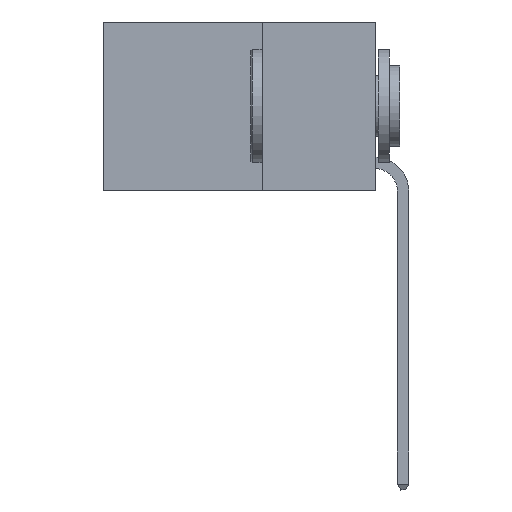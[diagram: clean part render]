
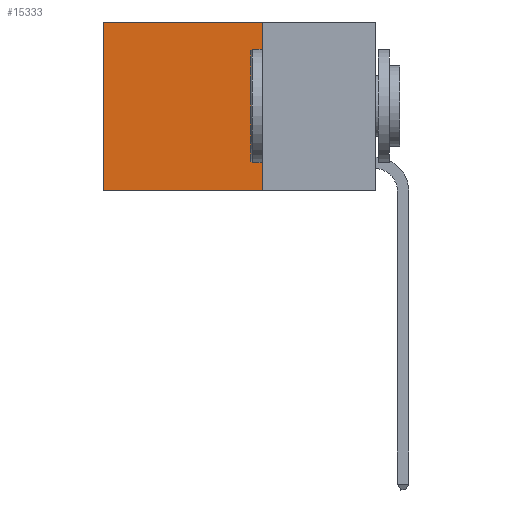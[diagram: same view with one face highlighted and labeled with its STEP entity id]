
A CAD part, left-side view. The second image highlights one B-rep face of the part: STEP entity #15333.
In plain terms, the highlighted planar face has unit normal (-1, 0, 0).
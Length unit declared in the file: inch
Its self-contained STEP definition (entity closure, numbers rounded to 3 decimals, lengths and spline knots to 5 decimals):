
#120 = EDGE_CURVE ( 'NONE', #6034, #5450, #17136, .T. ) ;
#121 = CARTESIAN_POINT ( 'NONE',  ( 0.2625, 0.25, 0. ) ) ;
#927 = CARTESIAN_POINT ( 'NONE',  ( 0.2625, 0.6, 0. ) ) ;
#1269 = EDGE_CURVE ( 'NONE', #15611, #5450, #10106, .T. ) ;
#1338 = EDGE_LOOP ( 'NONE', ( #2834, #15156, #6869, #9837 ) ) ;
#2278 = DIRECTION ( 'NONE',  ( 0., 0., -1. ) ) ;
#2834 = ORIENTED_EDGE ( 'NONE', *, *, #1269, .T. ) ;
#3060 = DIRECTION ( 'NONE',  ( 0., 1., 0. ) ) ;
#5450 = VERTEX_POINT ( 'NONE', #12162 ) ;
#6034 = VERTEX_POINT ( 'NONE', #6337 ) ;
#6337 = CARTESIAN_POINT ( 'NONE',  ( 0.2625, 0.25, -0.37 ) ) ;
#6578 = DIRECTION ( 'NONE',  ( 0., 1., 0. ) ) ;
#6858 = PLANE ( 'NONE',  #10512 ) ;
#6869 = ORIENTED_EDGE ( 'NONE', *, *, #15354, .F. ) ;
#7106 = DIRECTION ( 'NONE',  ( 0., 0., -1. ) ) ;
#7908 = LINE ( 'NONE', #121, #19855 ) ;
#8640 = CARTESIAN_POINT ( 'NONE',  ( 0.2625, 0.25, 0. ) ) ;
#8798 = EDGE_CURVE ( 'NONE', #13534, #15611, #15062, .T. ) ;
#8818 = CARTESIAN_POINT ( 'NONE',  ( 0.2625, 0.25, 0. ) ) ;
#9479 = CARTESIAN_POINT ( 'NONE',  ( 0.2625, 0.25, 0. ) ) ;
#9837 = ORIENTED_EDGE ( 'NONE', *, *, #8798, .T. ) ;
#10106 = LINE ( 'NONE', #927, #10547 ) ;
#10512 = AXIS2_PLACEMENT_3D ( 'NONE', #8640, #19147, #2278 ) ;
#10547 = VECTOR ( 'NONE', #7106, 39.37008 ) ;
#10916 = DIRECTION ( 'NONE',  ( 0., 0., -1. ) ) ;
#12162 = CARTESIAN_POINT ( 'NONE',  ( 0.2625, 0.6, -0.37 ) ) ;
#13534 = VERTEX_POINT ( 'NONE', #9479 ) ;
#14214 = CARTESIAN_POINT ( 'NONE',  ( 0.2625, 0.25, -0.37 ) ) ;
#15062 = LINE ( 'NONE', #8818, #17846 ) ;
#15156 = ORIENTED_EDGE ( 'NONE', *, *, #120, .F. ) ;
#15333 = ADVANCED_FACE ( 'NONE', ( #16087 ), #6858, .F. ) ;
#15354 = EDGE_CURVE ( 'NONE', #13534, #6034, #7908, .T. ) ;
#15611 = VERTEX_POINT ( 'NONE', #17776 ) ;
#15845 = VECTOR ( 'NONE', #6578, 39.37008 ) ;
#16087 = FACE_OUTER_BOUND ( 'NONE', #1338, .T. ) ;
#17136 = LINE ( 'NONE', #14214, #15845 ) ;
#17776 = CARTESIAN_POINT ( 'NONE',  ( 0.2625, 0.6, 0. ) ) ;
#17846 = VECTOR ( 'NONE', #3060, 39.37008 ) ;
#19147 = DIRECTION ( 'NONE',  ( 1., 0., 0. ) ) ;
#19855 = VECTOR ( 'NONE', #10916, 39.37008 ) ;
